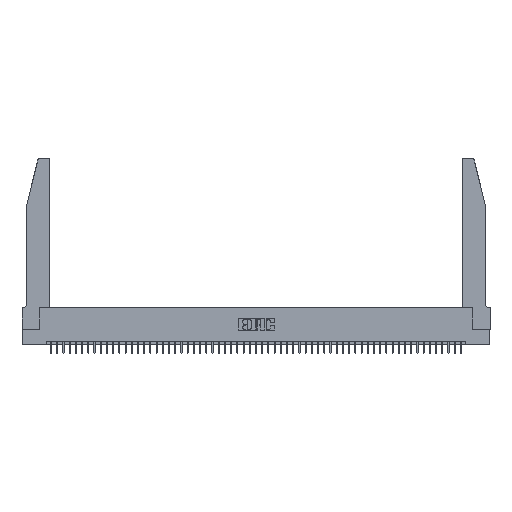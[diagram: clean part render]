
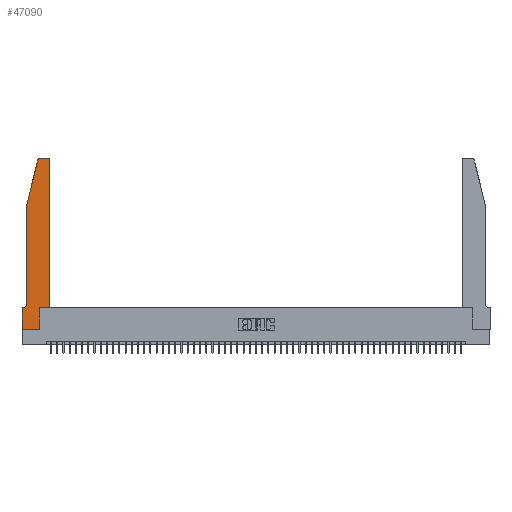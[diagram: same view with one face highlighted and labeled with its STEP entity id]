
A CAD part, top view. The second image highlights one B-rep face of the part: STEP entity #47090.
In plain terms, the highlighted planar face has unit normal (0, 0, 1).
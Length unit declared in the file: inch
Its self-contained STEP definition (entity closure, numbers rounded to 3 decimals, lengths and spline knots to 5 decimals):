
#260 = EDGE_CURVE ( 'NONE', #32338, #41256, #32262, .T. ) ;
#635 = VERTEX_POINT ( 'NONE', #15800 ) ;
#1101 = VERTEX_POINT ( 'NONE', #48773 ) ;
#1287 = DIRECTION ( 'NONE',  ( -1., 0., 0. ) ) ;
#2225 = LINE ( 'NONE', #32032, #11926 ) ;
#2426 = CARTESIAN_POINT ( 'NONE',  ( 0.0755, 0.35, 0.37 ) ) ;
#3151 = VECTOR ( 'NONE', #37009, 39.37008 ) ;
#3643 = LINE ( 'NONE', #36481, #3151 ) ;
#4080 = CARTESIAN_POINT ( 'NONE',  ( 0.2865, 0., 0.37 ) ) ;
#5032 = DIRECTION ( 'NONE',  ( 1., 0., 0. ) ) ;
#5503 = EDGE_CURVE ( 'NONE', #51516, #53105, #26293, .T. ) ;
#5748 = ORIENTED_EDGE ( 'NONE', *, *, #11341, .T. ) ;
#5836 = DIRECTION ( 'NONE',  ( 1., 0., 0. ) ) ;
#7316 = DIRECTION ( 'NONE',  ( 0., 0., 1. ) ) ;
#7347 = LINE ( 'NONE', #52501, #15794 ) ;
#7657 = VERTEX_POINT ( 'NONE', #44361 ) ;
#8522 = ORIENTED_EDGE ( 'NONE', *, *, #39654, .T. ) ;
#9136 = CARTESIAN_POINT ( 'NONE',  ( 0., 0., 0.37 ) ) ;
#10164 = ORIENTED_EDGE ( 'NONE', *, *, #17423, .T. ) ;
#10449 = EDGE_CURVE ( 'NONE', #1101, #32338, #34548, .T. ) ;
#10598 = DIRECTION ( 'NONE',  ( 1., 0., 0. ) ) ;
#11264 = DIRECTION ( 'NONE',  ( -0.239, -0.971, 0. ) ) ;
#11304 = CARTESIAN_POINT ( 'NONE',  ( 0.284, 2.75, 0.37 ) ) ;
#11341 = EDGE_CURVE ( 'NONE', #27168, #46775, #13354, .T. ) ;
#11356 = CARTESIAN_POINT ( 'NONE',  ( 0.0055, 0.35, 0.37 ) ) ;
#11424 = ORIENTED_EDGE ( 'NONE', *, *, #10449, .T. ) ;
#11497 = CARTESIAN_POINT ( 'NONE',  ( 0.2865, 0.35, 0.37 ) ) ;
#11926 = VECTOR ( 'NONE', #11264, 39.37008 ) ;
#12198 = CARTESIAN_POINT ( 'NONE',  ( 0., 0.35, 0.37 ) ) ;
#12561 = CARTESIAN_POINT ( 'NONE',  ( 0.2865, 0.35, 0.37 ) ) ;
#13354 = CIRCLE ( 'NONE', #27306, 0.07 ) ;
#13726 = CIRCLE ( 'NONE', #44304, 0.03 ) ;
#14093 = CARTESIAN_POINT ( 'NONE',  ( 0.25487, 2.72718, 0.37 ) ) ;
#14409 = DIRECTION ( 'NONE',  ( 0., 0., 1. ) ) ;
#14640 = EDGE_LOOP ( 'NONE', ( #39768, #17878, #10164, #23077, #5748, #41760, #8522, #11424, #38965, #14649, #50643, #21072 ) ) ;
#14649 = ORIENTED_EDGE ( 'NONE', *, *, #38366, .T. ) ;
#15004 = DIRECTION ( 'NONE',  ( 0., -1., 0. ) ) ;
#15157 = CARTESIAN_POINT ( 'NONE',  ( 0., 0., 0.37 ) ) ;
#15447 = VERTEX_POINT ( 'NONE', #12198 ) ;
#15794 = VECTOR ( 'NONE', #15004, 39.37008 ) ;
#15800 = CARTESIAN_POINT ( 'NONE',  ( 0.4505, 2.72, 0.37 ) ) ;
#15839 = DIRECTION ( 'NONE',  ( -1., 0., 0. ) ) ;
#15959 = CARTESIAN_POINT ( 'NONE',  ( 0.4505, 0.35, 0.37 ) ) ;
#16106 = LINE ( 'NONE', #2426, #46030 ) ;
#16231 = DIRECTION ( 'NONE',  ( 1., 0., 0. ) ) ;
#17423 = EDGE_CURVE ( 'NONE', #53105, #42726, #2225, .T. ) ;
#17878 = ORIENTED_EDGE ( 'NONE', *, *, #5503, .T. ) ;
#18488 = DIRECTION ( 'NONE',  ( 1., 0., 0. ) ) ;
#19725 = VECTOR ( 'NONE', #46976, 39.37008 ) ;
#21072 = ORIENTED_EDGE ( 'NONE', *, *, #40305, .T. ) ;
#21961 = DIRECTION ( 'NONE',  ( -1., 0., 0. ) ) ;
#22497 = LINE ( 'NONE', #50457, #41766 ) ;
#23077 = ORIENTED_EDGE ( 'NONE', *, *, #35241, .T. ) ;
#24665 = VECTOR ( 'NONE', #31712, 39.37008 ) ;
#24758 = VECTOR ( 'NONE', #16231, 39.37008 ) ;
#25920 = EDGE_CURVE ( 'NONE', #41637, #635, #3643, .T. ) ;
#26226 = EDGE_CURVE ( 'NONE', #46775, #15447, #16106, .T. ) ;
#26293 = CIRCLE ( 'NONE', #34915, 0.03 ) ;
#27069 = CARTESIAN_POINT ( 'NONE',  ( 0.0755, 2., 0.37 ) ) ;
#27168 = VERTEX_POINT ( 'NONE', #47119 ) ;
#27306 = AXIS2_PLACEMENT_3D ( 'NONE', #47777, #38749, #1287 ) ;
#30542 = CARTESIAN_POINT ( 'NONE',  ( 0.284, 2.72, 0.37 ) ) ;
#30694 = AXIS2_PLACEMENT_3D ( 'NONE', #50726, #43310, #5836 ) ;
#31712 = DIRECTION ( 'NONE',  ( 0., 1., 0. ) ) ;
#32032 = CARTESIAN_POINT ( 'NONE',  ( 0.0755, 2., 0.37 ) ) ;
#32262 = LINE ( 'NONE', #11497, #24665 ) ;
#32338 = VERTEX_POINT ( 'NONE', #4080 ) ;
#34548 = LINE ( 'NONE', #9136, #46827 ) ;
#34915 = AXIS2_PLACEMENT_3D ( 'NONE', #30542, #14409, #18488 ) ;
#35241 = EDGE_CURVE ( 'NONE', #42726, #27168, #7347, .T. ) ;
#36481 = CARTESIAN_POINT ( 'NONE',  ( 0.4505, 0.35, 0.37 ) ) ;
#37009 = DIRECTION ( 'NONE',  ( 0., 1., 0. ) ) ;
#38366 = EDGE_CURVE ( 'NONE', #41256, #41637, #49885, .T. ) ;
#38749 = DIRECTION ( 'NONE',  ( 0., 0., -1. ) ) ;
#38965 = ORIENTED_EDGE ( 'NONE', *, *, #260, .T. ) ;
#39654 = EDGE_CURVE ( 'NONE', #15447, #1101, #40041, .T. ) ;
#39768 = ORIENTED_EDGE ( 'NONE', *, *, #41004, .T. ) ;
#40041 = LINE ( 'NONE', #15157, #19725 ) ;
#40305 = EDGE_CURVE ( 'NONE', #635, #7657, #13726, .T. ) ;
#41004 = EDGE_CURVE ( 'NONE', #7657, #51516, #22497, .T. ) ;
#41256 = VERTEX_POINT ( 'NONE', #12561 ) ;
#41637 = VERTEX_POINT ( 'NONE', #43369 ) ;
#41760 = ORIENTED_EDGE ( 'NONE', *, *, #26226, .T. ) ;
#41766 = VECTOR ( 'NONE', #21961, 39.37008 ) ;
#42726 = VERTEX_POINT ( 'NONE', #27069 ) ;
#42761 = FACE_OUTER_BOUND ( 'NONE', #14640, .T. ) ;
#43310 = DIRECTION ( 'NONE',  ( 0., 0., 1. ) ) ;
#43369 = CARTESIAN_POINT ( 'NONE',  ( 0.4505, 0.35, 0.37 ) ) ;
#44304 = AXIS2_PLACEMENT_3D ( 'NONE', #48054, #7316, #10598 ) ;
#44361 = CARTESIAN_POINT ( 'NONE',  ( 0.4205, 2.75, 0.37 ) ) ;
#46030 = VECTOR ( 'NONE', #15839, 39.37008 ) ;
#46775 = VERTEX_POINT ( 'NONE', #11356 ) ;
#46827 = VECTOR ( 'NONE', #5032, 39.37008 ) ;
#46976 = DIRECTION ( 'NONE',  ( 0., -1., 0. ) ) ;
#47090 = ADVANCED_FACE ( 'NONE', ( #42761 ), #51552, .T. ) ;
#47119 = CARTESIAN_POINT ( 'NONE',  ( 0.0755, 0.42, 0.37 ) ) ;
#47777 = CARTESIAN_POINT ( 'NONE',  ( 0.0055, 0.42, 0.37 ) ) ;
#48054 = CARTESIAN_POINT ( 'NONE',  ( 0.4205, 2.72, 0.37 ) ) ;
#48773 = CARTESIAN_POINT ( 'NONE',  ( 0., 0., 0.37 ) ) ;
#49885 = LINE ( 'NONE', #15959, #24758 ) ;
#50457 = CARTESIAN_POINT ( 'NONE',  ( 0.2605, 2.75, 0.37 ) ) ;
#50643 = ORIENTED_EDGE ( 'NONE', *, *, #25920, .T. ) ;
#50726 = CARTESIAN_POINT ( 'NONE',  ( 0., 0.35, 0.37 ) ) ;
#51516 = VERTEX_POINT ( 'NONE', #11304 ) ;
#51552 = PLANE ( 'NONE',  #30694 ) ;
#52501 = CARTESIAN_POINT ( 'NONE',  ( 0.0755, 2., 0.37 ) ) ;
#53105 = VERTEX_POINT ( 'NONE', #14093 ) ;
